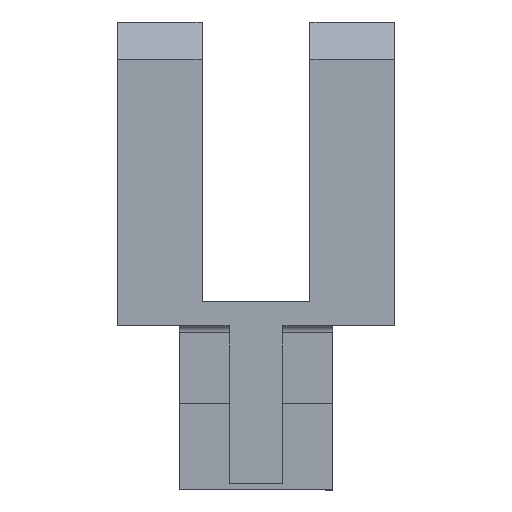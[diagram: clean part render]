
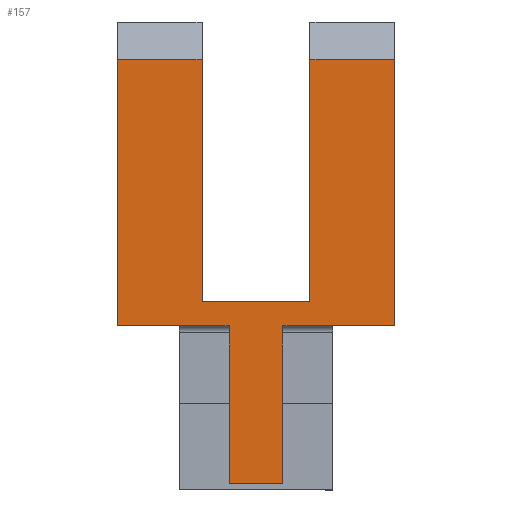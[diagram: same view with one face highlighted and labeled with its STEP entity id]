
A CAD part, front view. The second image highlights one B-rep face of the part: STEP entity #157.
In plain terms, the highlighted planar face has unit normal (0, -1, 0).
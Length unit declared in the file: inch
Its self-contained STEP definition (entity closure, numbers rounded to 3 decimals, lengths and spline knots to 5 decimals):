
#8 = CARTESIAN_POINT ( 'NONE',  ( 1.365, -0.5, 5.4 ) ) ;
#33 = EDGE_CURVE ( 'NONE', #504, #2168, #1066, .T. ) ;
#44 = CARTESIAN_POINT ( 'NONE',  ( 0., -0.5, 5.4 ) ) ;
#88 = ORIENTED_EDGE ( 'NONE', *, *, #2346, .T. ) ;
#119 = VERTEX_POINT ( 'NONE', #224 ) ;
#157 = ADVANCED_FACE ( 'NONE', ( #725 ), #2613, .T. ) ;
#224 = CARTESIAN_POINT ( 'NONE',  ( 1.8, -0.5, 1.1 ) ) ;
#254 = ORIENTED_EDGE ( 'NONE', *, *, #2151, .T. ) ;
#253 = DIRECTION ( 'NONE',  ( -1., 0., 0. ) ) ;
#344 = CARTESIAN_POINT ( 'NONE',  ( 0., -0.5, 5.4 ) ) ;
#353 = EDGE_CURVE ( 'NONE', #1175, #2063, #1063, .T. ) ;
#425 = LINE ( 'NONE', #2222, #2656 ) ;
#439 = EDGE_LOOP ( 'NONE', ( #533, #2684, #1915, #88, #744, #2597, #1142, #1358, #643, #2757, #1483, #254 ) ) ;
#459 = CARTESIAN_POINT ( 'NONE',  ( 3.105, -0.5, 5.4 ) ) ;
#482 = CARTESIAN_POINT ( 'NONE',  ( 0., -0.5, 1.5 ) ) ;
#504 = VERTEX_POINT ( 'NONE', #344 ) ;
#527 = DIRECTION ( 'NONE',  ( 0., 0., -1. ) ) ;
#533 = ORIENTED_EDGE ( 'NONE', *, *, #353, .T. ) ;
#535 = CARTESIAN_POINT ( 'NONE',  ( 0., -0.5, 1.1 ) ) ;
#547 = CARTESIAN_POINT ( 'NONE',  ( 2.67, -0.5, -1.44614 ) ) ;
#643 = ORIENTED_EDGE ( 'NONE', *, *, #1127, .T. ) ;
#655 = VECTOR ( 'NONE', #2686, 39.37008 ) ;
#665 = CARTESIAN_POINT ( 'NONE',  ( 0., -0.5, 0. ) ) ;
#679 = VECTOR ( 'NONE', #865, 39.37008 ) ;
#708 = DIRECTION ( 'NONE',  ( 0., 0., 1. ) ) ;
#715 = VECTOR ( 'NONE', #253, 39.37008 ) ;
#725 = FACE_OUTER_BOUND ( 'NONE', #439, .T. ) ;
#744 = ORIENTED_EDGE ( 'NONE', *, *, #1325, .T. ) ;
#861 = EDGE_CURVE ( 'NONE', #1597, #2380, #2093, .T. ) ;
#865 = DIRECTION ( 'NONE',  ( 0., 0., -1. ) ) ;
#869 = LINE ( 'NONE', #459, #1075 ) ;
#914 = DIRECTION ( 'NONE',  ( 0., 0., -1. ) ) ;
#1000 = LINE ( 'NONE', #2557, #1895 ) ;
#1006 = EDGE_CURVE ( 'NONE', #2063, #504, #1058, .T. ) ;
#1016 = DIRECTION ( 'NONE',  ( 0., 0., 1. ) ) ;
#1058 = LINE ( 'NONE', #44, #715 ) ;
#1063 = LINE ( 'NONE', #1171, #1428 ) ;
#1066 = LINE ( 'NONE', #2128, #679 ) ;
#1075 = VECTOR ( 'NONE', #1988, 39.37008 ) ;
#1076 = EDGE_CURVE ( 'NONE', #1515, #2330, #425, .T. ) ;
#1127 = EDGE_CURVE ( 'NONE', #1505, #2612, #2493, .T. ) ;
#1129 = DIRECTION ( 'NONE',  ( 0., 0., 1. ) ) ;
#1142 = ORIENTED_EDGE ( 'NONE', *, *, #861, .T. ) ;
#1171 = CARTESIAN_POINT ( 'NONE',  ( 1.365, -0.5, 0. ) ) ;
#1172 = CARTESIAN_POINT ( 'NONE',  ( 2.67, -0.5, -1.44614 ) ) ;
#1175 = VERTEX_POINT ( 'NONE', #2655 ) ;
#1207 = LINE ( 'NONE', #547, #655 ) ;
#1246 = VECTOR ( 'NONE', #2190, 39.37008 ) ;
#1312 = LINE ( 'NONE', #482, #1246 ) ;
#1325 = EDGE_CURVE ( 'NONE', #119, #2170, #1000, .T. ) ;
#1330 = CARTESIAN_POINT ( 'NONE',  ( 0., -0.5, 1.1 ) ) ;
#1335 = DIRECTION ( 'NONE',  ( 0., -1., 0. ) ) ;
#1358 = ORIENTED_EDGE ( 'NONE', *, *, #2756, .T. ) ;
#1424 = CARTESIAN_POINT ( 'NONE',  ( 0., -0.5, 1.1 ) ) ;
#1428 = VECTOR ( 'NONE', #1016, 39.37008 ) ;
#1462 = VECTOR ( 'NONE', #1129, 39.37008 ) ;
#1477 = LINE ( 'NONE', #1424, #2745 ) ;
#1483 = ORIENTED_EDGE ( 'NONE', *, *, #1076, .T. ) ;
#1505 = VERTEX_POINT ( 'NONE', #2225 ) ;
#1515 = VERTEX_POINT ( 'NONE', #2436 ) ;
#1597 = VERTEX_POINT ( 'NONE', #2659 ) ;
#1621 = EDGE_CURVE ( 'NONE', #2170, #1597, #1207, .T. ) ;
#1737 = VECTOR ( 'NONE', #2427, 39.37008 ) ;
#1740 = CARTESIAN_POINT ( 'NONE',  ( 1.8, -0.5, -1.44614 ) ) ;
#1788 = VECTOR ( 'NONE', #708, 39.37008 ) ;
#1871 = LINE ( 'NONE', #1330, #1737 ) ;
#1895 = VECTOR ( 'NONE', #2781, 39.37008 ) ;
#1915 = ORIENTED_EDGE ( 'NONE', *, *, #33, .T. ) ;
#1988 = DIRECTION ( 'NONE',  ( -1., 0., 0. ) ) ;
#2063 = VERTEX_POINT ( 'NONE', #8 ) ;
#2093 = LINE ( 'NONE', #1172, #1462 ) ;
#2128 = CARTESIAN_POINT ( 'NONE',  ( 0., -0.5, 0. ) ) ;
#2151 = EDGE_CURVE ( 'NONE', #2330, #1175, #1312, .T. ) ;
#2168 = VERTEX_POINT ( 'NONE', #535 ) ;
#2170 = VERTEX_POINT ( 'NONE', #1740 ) ;
#2190 = DIRECTION ( 'NONE',  ( -1., 0., 0. ) ) ;
#2222 = CARTESIAN_POINT ( 'NONE',  ( 3.105, -0.5, 0. ) ) ;
#2225 = CARTESIAN_POINT ( 'NONE',  ( 4.47, -0.5, 1.1 ) ) ;
#2268 = CARTESIAN_POINT ( 'NONE',  ( 3.105, -0.5, 1.5 ) ) ;
#2295 = CARTESIAN_POINT ( 'NONE',  ( 2.67, -0.5, 1.1 ) ) ;
#2330 = VERTEX_POINT ( 'NONE', #2268 ) ;
#2346 = EDGE_CURVE ( 'NONE', #2168, #119, #1477, .T. ) ;
#2369 = AXIS2_PLACEMENT_3D ( 'NONE', #665, #1335, #914 ) ;
#2380 = VERTEX_POINT ( 'NONE', #2295 ) ;
#2427 = DIRECTION ( 'NONE',  ( 1., 0., 0. ) ) ;
#2436 = CARTESIAN_POINT ( 'NONE',  ( 3.105, -0.5, 5.4 ) ) ;
#2490 = DIRECTION ( 'NONE',  ( 1., 0., 0. ) ) ;
#2493 = LINE ( 'NONE', #2645, #1788 ) ;
#2557 = CARTESIAN_POINT ( 'NONE',  ( 1.8, -0.5, -1.44614 ) ) ;
#2597 = ORIENTED_EDGE ( 'NONE', *, *, #1621, .T. ) ;
#2612 = VERTEX_POINT ( 'NONE', #2784 ) ;
#2613 = PLANE ( 'NONE',  #2369 ) ;
#2645 = CARTESIAN_POINT ( 'NONE',  ( 4.47, -0.5, 0. ) ) ;
#2655 = CARTESIAN_POINT ( 'NONE',  ( 1.365, -0.5, 1.5 ) ) ;
#2656 = VECTOR ( 'NONE', #527, 39.37008 ) ;
#2659 = CARTESIAN_POINT ( 'NONE',  ( 2.67, -0.5, -1.44614 ) ) ;
#2684 = ORIENTED_EDGE ( 'NONE', *, *, #1006, .T. ) ;
#2686 = DIRECTION ( 'NONE',  ( 1., 0., 0. ) ) ;
#2718 = EDGE_CURVE ( 'NONE', #2612, #1515, #869, .T. ) ;
#2745 = VECTOR ( 'NONE', #2490, 39.37008 ) ;
#2756 = EDGE_CURVE ( 'NONE', #2380, #1505, #1871, .T. ) ;
#2757 = ORIENTED_EDGE ( 'NONE', *, *, #2718, .T. ) ;
#2781 = DIRECTION ( 'NONE',  ( 0., 0., -1. ) ) ;
#2784 = CARTESIAN_POINT ( 'NONE',  ( 4.47, -0.5, 5.4 ) ) ;
